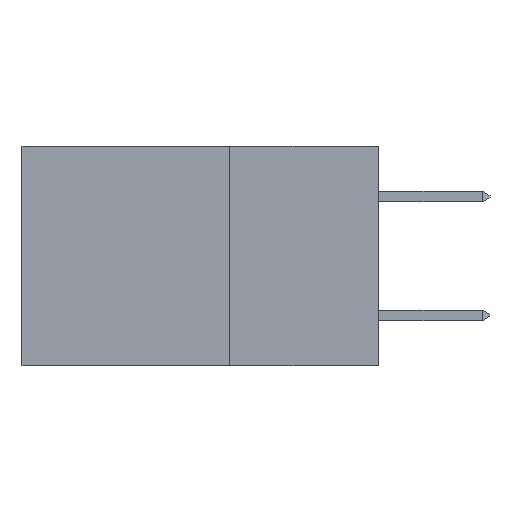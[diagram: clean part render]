
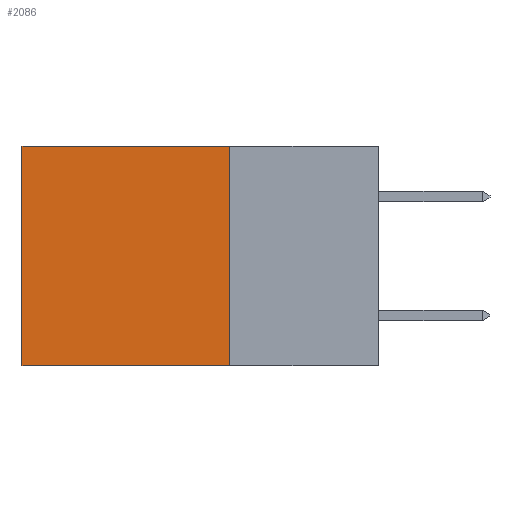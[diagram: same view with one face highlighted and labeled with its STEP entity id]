
A CAD part, left-side view. The second image highlights one B-rep face of the part: STEP entity #2086.
In plain terms, the highlighted planar face has unit normal (-1, 0, 0).
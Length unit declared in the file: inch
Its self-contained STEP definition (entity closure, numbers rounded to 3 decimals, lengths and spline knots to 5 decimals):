
#540 = CARTESIAN_POINT ( 'NONE',  ( 0.298, 0.25, 0. ) ) ;
#1156 = CARTESIAN_POINT ( 'NONE',  ( 0.298, 0.25, -0.37 ) ) ;
#1250 = DIRECTION ( 'NONE',  ( 0., 0., -1. ) ) ;
#1398 = CARTESIAN_POINT ( 'NONE',  ( 0.298, 0.25, -0.37 ) ) ;
#1842 = LINE ( 'NONE', #6324, #4543 ) ;
#2086 = ADVANCED_FACE ( 'NONE', ( #6251 ), #6029, .F. ) ;
#2563 = VERTEX_POINT ( 'NONE', #3155 ) ;
#2592 = CARTESIAN_POINT ( 'NONE',  ( 0.298, 0.25, 0. ) ) ;
#2866 = ORIENTED_EDGE ( 'NONE', *, *, #7639, .T. ) ;
#2998 = AXIS2_PLACEMENT_3D ( 'NONE', #9639, #8606, #6998 ) ;
#3155 = CARTESIAN_POINT ( 'NONE',  ( 0.298, 0.6, 0. ) ) ;
#3437 = LINE ( 'NONE', #2592, #8279 ) ;
#3514 = VECTOR ( 'NONE', #8986, 39.37008 ) ;
#3975 = VERTEX_POINT ( 'NONE', #540 ) ;
#4543 = VECTOR ( 'NONE', #6298, 39.37008 ) ;
#5045 = ORIENTED_EDGE ( 'NONE', *, *, #6550, .F. ) ;
#5504 = ORIENTED_EDGE ( 'NONE', *, *, #10535, .F. ) ;
#5618 = VERTEX_POINT ( 'NONE', #7000 ) ;
#5952 = VECTOR ( 'NONE', #1250, 39.37008 ) ;
#6029 = PLANE ( 'NONE',  #2998 ) ;
#6251 = FACE_OUTER_BOUND ( 'NONE', #11558, .T. ) ;
#6298 = DIRECTION ( 'NONE',  ( 0., 0., -1. ) ) ;
#6324 = CARTESIAN_POINT ( 'NONE',  ( 0.298, 0.25, 0. ) ) ;
#6550 = EDGE_CURVE ( 'NONE', #3975, #12556, #1842, .T. ) ;
#6998 = DIRECTION ( 'NONE',  ( 0., 0., -1. ) ) ;
#7000 = CARTESIAN_POINT ( 'NONE',  ( 0.298, 0.6, -0.37 ) ) ;
#7639 = EDGE_CURVE ( 'NONE', #3975, #2563, #3437, .T. ) ;
#8063 = EDGE_CURVE ( 'NONE', #2563, #5618, #8591, .T. ) ;
#8279 = VECTOR ( 'NONE', #8442, 39.37008 ) ;
#8442 = DIRECTION ( 'NONE',  ( 0., 1., 0. ) ) ;
#8591 = LINE ( 'NONE', #10985, #5952 ) ;
#8606 = DIRECTION ( 'NONE',  ( 1., 0., 0. ) ) ;
#8702 = ORIENTED_EDGE ( 'NONE', *, *, #8063, .T. ) ;
#8986 = DIRECTION ( 'NONE',  ( 0., 1., 0. ) ) ;
#9639 = CARTESIAN_POINT ( 'NONE',  ( 0.298, 0.25, 0. ) ) ;
#10535 = EDGE_CURVE ( 'NONE', #12556, #5618, #11195, .T. ) ;
#10985 = CARTESIAN_POINT ( 'NONE',  ( 0.298, 0.6, 0. ) ) ;
#11195 = LINE ( 'NONE', #1156, #3514 ) ;
#11558 = EDGE_LOOP ( 'NONE', ( #8702, #5504, #5045, #2866 ) ) ;
#12556 = VERTEX_POINT ( 'NONE', #1398 ) ;
